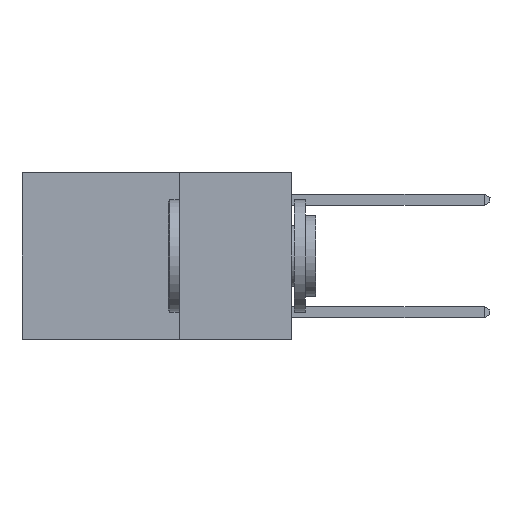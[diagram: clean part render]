
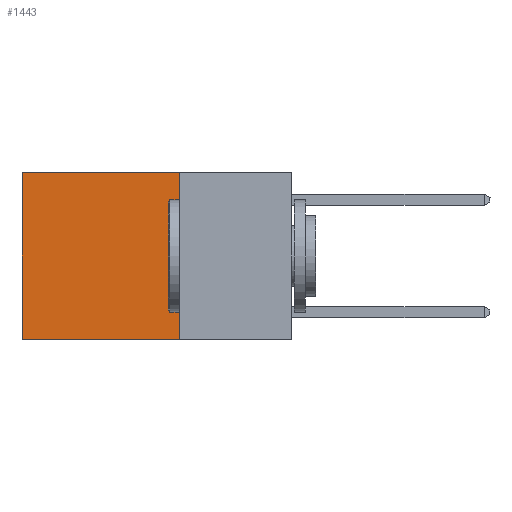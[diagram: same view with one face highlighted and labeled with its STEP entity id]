
A CAD part, left-side view. The second image highlights one B-rep face of the part: STEP entity #1443.
In plain terms, the highlighted planar face has unit normal (-1, 0, 0).
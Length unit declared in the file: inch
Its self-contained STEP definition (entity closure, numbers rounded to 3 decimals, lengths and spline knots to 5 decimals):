
#581 = DIRECTION ( 'NONE',  ( 0., 0., -1. ) ) ;
#857 = CARTESIAN_POINT ( 'NONE',  ( 0.2625, 0.6, -0.37 ) ) ;
#1443 = ADVANCED_FACE ( 'NONE', ( #3427 ), #3688, .F. ) ;
#1487 = CARTESIAN_POINT ( 'NONE',  ( 0.2625, 0.25, 0. ) ) ;
#1880 = DIRECTION ( 'NONE',  ( 0., 1., 0. ) ) ;
#2379 = ORIENTED_EDGE ( 'NONE', *, *, #13042, .F. ) ;
#3427 = FACE_OUTER_BOUND ( 'NONE', #7644, .T. ) ;
#3688 = PLANE ( 'NONE',  #21480 ) ;
#3820 = CARTESIAN_POINT ( 'NONE',  ( 0.2625, 0.25, 0. ) ) ;
#4347 = ORIENTED_EDGE ( 'NONE', *, *, #15746, .T. ) ;
#4356 = LINE ( 'NONE', #19911, #18424 ) ;
#4576 = EDGE_CURVE ( 'NONE', #17105, #12460, #4356, .T. ) ;
#4699 = ORIENTED_EDGE ( 'NONE', *, *, #23011, .T. ) ;
#5892 = DIRECTION ( 'NONE',  ( 0., 1., 0. ) ) ;
#6616 = VERTEX_POINT ( 'NONE', #857 ) ;
#7644 = EDGE_LOOP ( 'NONE', ( #4699, #2379, #15277, #4347 ) ) ;
#7882 = DIRECTION ( 'NONE',  ( 0., 0., -1. ) ) ;
#10455 = VECTOR ( 'NONE', #1880, 39.37008 ) ;
#11378 = LINE ( 'NONE', #13182, #10455 ) ;
#12460 = VERTEX_POINT ( 'NONE', #15143 ) ;
#13042 = EDGE_CURVE ( 'NONE', #12460, #6616, #11378, .T. ) ;
#13182 = CARTESIAN_POINT ( 'NONE',  ( 0.2625, 0.25, -0.37 ) ) ;
#13249 = CARTESIAN_POINT ( 'NONE',  ( 0.2625, 0.6, 0. ) ) ;
#13700 = LINE ( 'NONE', #21835, #16753 ) ;
#14042 = LINE ( 'NONE', #19978, #14185 ) ;
#14185 = VECTOR ( 'NONE', #7882, 39.37008 ) ;
#15143 = CARTESIAN_POINT ( 'NONE',  ( 0.2625, 0.25, -0.37 ) ) ;
#15277 = ORIENTED_EDGE ( 'NONE', *, *, #4576, .F. ) ;
#15746 = EDGE_CURVE ( 'NONE', #17105, #16463, #13700, .T. ) ;
#16463 = VERTEX_POINT ( 'NONE', #13249 ) ;
#16753 = VECTOR ( 'NONE', #5892, 39.37008 ) ;
#17105 = VERTEX_POINT ( 'NONE', #3820 ) ;
#18424 = VECTOR ( 'NONE', #581, 39.37008 ) ;
#19911 = CARTESIAN_POINT ( 'NONE',  ( 0.2625, 0.25, 0. ) ) ;
#19978 = CARTESIAN_POINT ( 'NONE',  ( 0.2625, 0.6, 0. ) ) ;
#21480 = AXIS2_PLACEMENT_3D ( 'NONE', #1487, #22994, #25046 ) ;
#21835 = CARTESIAN_POINT ( 'NONE',  ( 0.2625, 0.25, 0. ) ) ;
#22994 = DIRECTION ( 'NONE',  ( 1., 0., 0. ) ) ;
#23011 = EDGE_CURVE ( 'NONE', #16463, #6616, #14042, .T. ) ;
#25046 = DIRECTION ( 'NONE',  ( 0., 0., -1. ) ) ;
